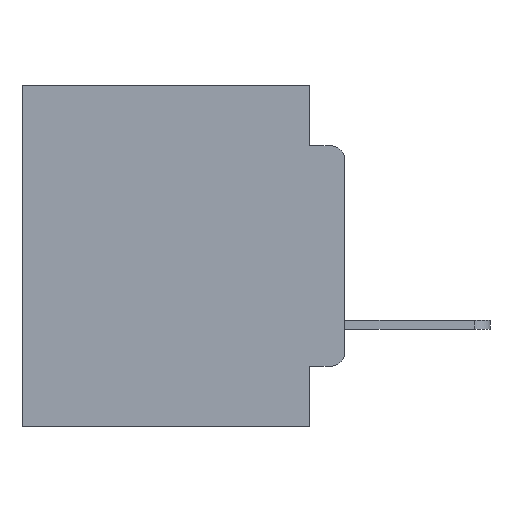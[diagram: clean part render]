
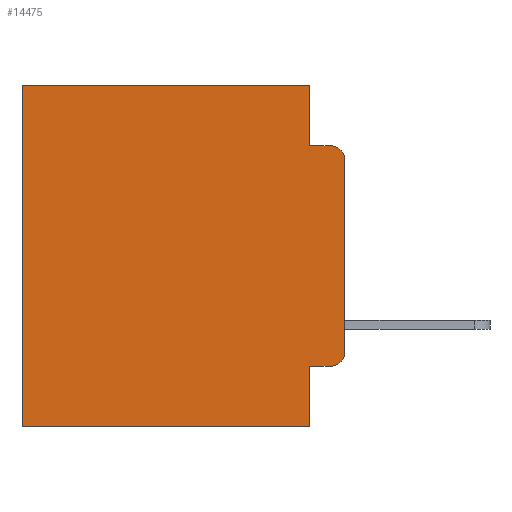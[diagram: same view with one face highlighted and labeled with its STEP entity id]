
A CAD part, left-side view. The second image highlights one B-rep face of the part: STEP entity #14475.
In plain terms, the highlighted planar face has unit normal (-1, 0, 0).
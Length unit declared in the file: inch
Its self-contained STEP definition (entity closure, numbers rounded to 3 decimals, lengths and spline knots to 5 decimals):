
#584 = CARTESIAN_POINT ( 'NONE',  ( 0.298, 0.02, -0.0885 ) ) ;
#926 = CARTESIAN_POINT ( 'NONE',  ( 0.298, 0.02, -0.4115 ) ) ;
#1005 = CIRCLE ( 'NONE', #4889, 0.02 ) ;
#1117 = CARTESIAN_POINT ( 'NONE',  ( 0.298, 0.051, -0.0885 ) ) ;
#1244 = CARTESIAN_POINT ( 'NONE',  ( 0.298, 0.051, 0. ) ) ;
#1846 = ORIENTED_EDGE ( 'NONE', *, *, #5425, .F. ) ;
#1911 = PLANE ( 'NONE',  #5097 ) ;
#2249 = CARTESIAN_POINT ( 'NONE',  ( 0.298, 0.051, 0. ) ) ;
#2398 = CARTESIAN_POINT ( 'NONE',  ( 0.298, 0.473, 0. ) ) ;
#2467 = EDGE_CURVE ( 'NONE', #25595, #26161, #10679, .T. ) ;
#2547 = VECTOR ( 'NONE', #17889, 39.37008 ) ;
#3190 = VECTOR ( 'NONE', #13686, 39.37008 ) ;
#3637 = EDGE_CURVE ( 'NONE', #8854, #22151, #18168, .T. ) ;
#3794 = VERTEX_POINT ( 'NONE', #1117 ) ;
#3875 = LINE ( 'NONE', #15978, #21608 ) ;
#4889 = AXIS2_PLACEMENT_3D ( 'NONE', #17334, #7186, #17590 ) ;
#5089 = CARTESIAN_POINT ( 'NONE',  ( 0.298, 0.473, 0. ) ) ;
#5097 = AXIS2_PLACEMENT_3D ( 'NONE', #17627, #7744, #23927 ) ;
#5219 = ORIENTED_EDGE ( 'NONE', *, *, #12991, .F. ) ;
#5231 = ORIENTED_EDGE ( 'NONE', *, *, #25840, .T. ) ;
#5417 = CIRCLE ( 'NONE', #15853, 0.02 ) ;
#5425 = EDGE_CURVE ( 'NONE', #11902, #20775, #3875, .T. ) ;
#5670 = CARTESIAN_POINT ( 'NONE',  ( 0.298, 0.02, -0.1085 ) ) ;
#5857 = DIRECTION ( 'NONE',  ( 0., 1., 0. ) ) ;
#6030 = VECTOR ( 'NONE', #7702, 39.37008 ) ;
#6126 = LINE ( 'NONE', #2398, #13712 ) ;
#6443 = VERTEX_POINT ( 'NONE', #12404 ) ;
#6650 = LINE ( 'NONE', #7493, #3190 ) ;
#6781 = CARTESIAN_POINT ( 'NONE',  ( 0.298, 0.051, 0. ) ) ;
#7186 = DIRECTION ( 'NONE',  ( -1., 0., 0. ) ) ;
#7465 = VERTEX_POINT ( 'NONE', #584 ) ;
#7493 = CARTESIAN_POINT ( 'NONE',  ( 0.298, 0., 0. ) ) ;
#7684 = DIRECTION ( 'NONE',  ( 0., 0., -1. ) ) ;
#7702 = DIRECTION ( 'NONE',  ( 0., 0., -1. ) ) ;
#7744 = DIRECTION ( 'NONE',  ( 1., 0., 0. ) ) ;
#8014 = VECTOR ( 'NONE', #10276, 39.37008 ) ;
#8196 = ORIENTED_EDGE ( 'NONE', *, *, #3637, .T. ) ;
#8762 = VECTOR ( 'NONE', #13180, 39.37008 ) ;
#8854 = VERTEX_POINT ( 'NONE', #6781 ) ;
#9074 = ORIENTED_EDGE ( 'NONE', *, *, #11882, .T. ) ;
#10276 = DIRECTION ( 'NONE',  ( 0., 0., -1. ) ) ;
#10568 = ORIENTED_EDGE ( 'NONE', *, *, #20190, .F. ) ;
#10679 = LINE ( 'NONE', #17129, #8762 ) ;
#11829 = LINE ( 'NONE', #2249, #8014 ) ;
#11882 = EDGE_CURVE ( 'NONE', #26161, #20347, #1005, .T. ) ;
#11902 = VERTEX_POINT ( 'NONE', #23380 ) ;
#12404 = CARTESIAN_POINT ( 'NONE',  ( 0.298, 0., -0.1085 ) ) ;
#12787 = CARTESIAN_POINT ( 'NONE',  ( 0.298, 0.051, -0.4115 ) ) ;
#12826 = EDGE_CURVE ( 'NONE', #6443, #20347, #6650, .T. ) ;
#12991 = EDGE_CURVE ( 'NONE', #3794, #7465, #23440, .T. ) ;
#13180 = DIRECTION ( 'NONE',  ( 0., -1., 0. ) ) ;
#13686 = DIRECTION ( 'NONE',  ( 0., 0., -1. ) ) ;
#13712 = VECTOR ( 'NONE', #24393, 39.37008 ) ;
#14475 = ADVANCED_FACE ( 'NONE', ( #16963 ), #1911, .F. ) ;
#15853 = AXIS2_PLACEMENT_3D ( 'NONE', #5670, #19778, #7684 ) ;
#15978 = CARTESIAN_POINT ( 'NONE',  ( 0.298, 0., -0.5 ) ) ;
#16057 = CARTESIAN_POINT ( 'NONE',  ( 0.298, 0., -0.3915 ) ) ;
#16425 = LINE ( 'NONE', #1244, #6030 ) ;
#16439 = ORIENTED_EDGE ( 'NONE', *, *, #2467, .T. ) ;
#16839 = ORIENTED_EDGE ( 'NONE', *, *, #18427, .T. ) ;
#16963 = FACE_OUTER_BOUND ( 'NONE', #17760, .T. ) ;
#17129 = CARTESIAN_POINT ( 'NONE',  ( 0.298, 0.051, -0.4115 ) ) ;
#17334 = CARTESIAN_POINT ( 'NONE',  ( 0.298, 0.02, -0.3915 ) ) ;
#17590 = DIRECTION ( 'NONE',  ( 0., 0., -1. ) ) ;
#17627 = CARTESIAN_POINT ( 'NONE',  ( 0.298, 0., 0. ) ) ;
#17760 = EDGE_LOOP ( 'NONE', ( #25087, #5231, #5219, #20402, #8196, #16839, #1846, #10568, #16439, #9074 ) ) ;
#17889 = DIRECTION ( 'NONE',  ( 0., -1., 0. ) ) ;
#18168 = LINE ( 'NONE', #24130, #23921 ) ;
#18427 = EDGE_CURVE ( 'NONE', #22151, #20775, #6126, .T. ) ;
#19778 = DIRECTION ( 'NONE',  ( -1., 0., 0. ) ) ;
#20099 = CARTESIAN_POINT ( 'NONE',  ( 0.298, 0.051, -0.0885 ) ) ;
#20190 = EDGE_CURVE ( 'NONE', #25595, #11902, #16425, .T. ) ;
#20347 = VERTEX_POINT ( 'NONE', #16057 ) ;
#20402 = ORIENTED_EDGE ( 'NONE', *, *, #24274, .F. ) ;
#20775 = VERTEX_POINT ( 'NONE', #23241 ) ;
#21608 = VECTOR ( 'NONE', #5857, 39.37008 ) ;
#22151 = VERTEX_POINT ( 'NONE', #5089 ) ;
#23241 = CARTESIAN_POINT ( 'NONE',  ( 0.298, 0.473, -0.5 ) ) ;
#23380 = CARTESIAN_POINT ( 'NONE',  ( 0.298, 0.051, -0.5 ) ) ;
#23440 = LINE ( 'NONE', #20099, #2547 ) ;
#23921 = VECTOR ( 'NONE', #26148, 39.37008 ) ;
#23927 = DIRECTION ( 'NONE',  ( 0., 0., -1. ) ) ;
#24130 = CARTESIAN_POINT ( 'NONE',  ( 0.298, 0., 0. ) ) ;
#24274 = EDGE_CURVE ( 'NONE', #8854, #3794, #11829, .T. ) ;
#24393 = DIRECTION ( 'NONE',  ( 0., 0., -1. ) ) ;
#25087 = ORIENTED_EDGE ( 'NONE', *, *, #12826, .F. ) ;
#25595 = VERTEX_POINT ( 'NONE', #12787 ) ;
#25840 = EDGE_CURVE ( 'NONE', #6443, #7465, #5417, .T. ) ;
#26148 = DIRECTION ( 'NONE',  ( 0., 1., 0. ) ) ;
#26161 = VERTEX_POINT ( 'NONE', #926 ) ;
